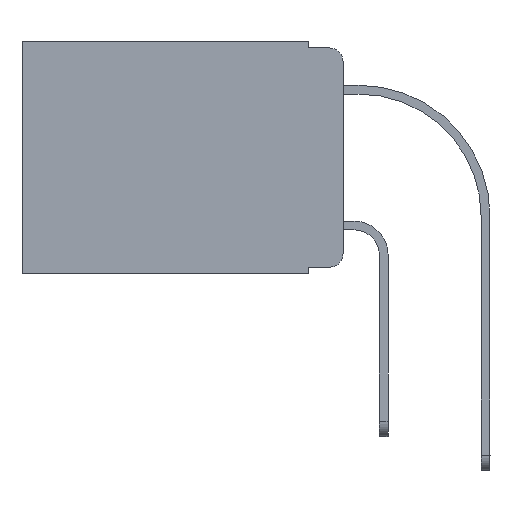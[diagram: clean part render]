
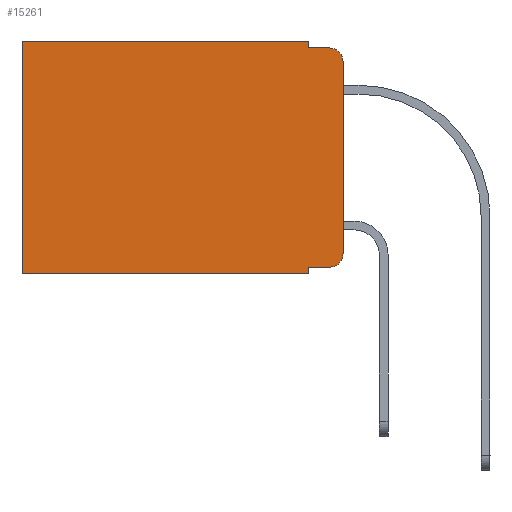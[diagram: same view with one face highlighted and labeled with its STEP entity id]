
A CAD part, left-side view. The second image highlights one B-rep face of the part: STEP entity #15261.
In plain terms, the highlighted planar face has unit normal (-1, 0, 0).
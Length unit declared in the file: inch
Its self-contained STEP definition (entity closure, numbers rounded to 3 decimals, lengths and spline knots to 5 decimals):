
#123 = CARTESIAN_POINT ( 'NONE',  ( 0.298, 0.02, -0.333 ) ) ;
#134 = CARTESIAN_POINT ( 'NONE',  ( 0.298, 0.051, -0.333 ) ) ;
#322 = CARTESIAN_POINT ( 'NONE',  ( 0.298, 0.051, -0.333 ) ) ;
#547 = VECTOR ( 'NONE', #4205, 39.37008 ) ;
#637 = EDGE_CURVE ( 'NONE', #14524, #1606, #16961, .T. ) ;
#685 = CARTESIAN_POINT ( 'NONE',  ( 0.298, 0.051, -0.01 ) ) ;
#919 = ORIENTED_EDGE ( 'NONE', *, *, #12089, .T. ) ;
#1377 = FACE_OUTER_BOUND ( 'NONE', #13782, .T. ) ;
#1388 = DIRECTION ( 'NONE',  ( 0., 0., -1. ) ) ;
#1590 = AXIS2_PLACEMENT_3D ( 'NONE', #2081, #9486, #15052 ) ;
#1606 = VERTEX_POINT ( 'NONE', #2224 ) ;
#1702 = CARTESIAN_POINT ( 'NONE',  ( 0.298, 0., 0. ) ) ;
#1849 = DIRECTION ( 'NONE',  ( 0., 1., 0. ) ) ;
#2081 = CARTESIAN_POINT ( 'NONE',  ( 0.298, 0.02, -0.03 ) ) ;
#2224 = CARTESIAN_POINT ( 'NONE',  ( 0.298, 0., -0.313 ) ) ;
#2403 = CARTESIAN_POINT ( 'NONE',  ( 0.298, 0.051, -0.01 ) ) ;
#2492 = AXIS2_PLACEMENT_3D ( 'NONE', #12650, #8907, #14354 ) ;
#2554 = VERTEX_POINT ( 'NONE', #14505 ) ;
#2789 = CARTESIAN_POINT ( 'NONE',  ( 0.298, 0.051, -0.343 ) ) ;
#2972 = DIRECTION ( 'NONE',  ( 0., 0., -1. ) ) ;
#3544 = ORIENTED_EDGE ( 'NONE', *, *, #9030, .T. ) ;
#3619 = LINE ( 'NONE', #14890, #21005 ) ;
#4083 = LINE ( 'NONE', #322, #547 ) ;
#4205 = DIRECTION ( 'NONE',  ( 0., -1., 0. ) ) ;
#4498 = ORIENTED_EDGE ( 'NONE', *, *, #12221, .F. ) ;
#4610 = VECTOR ( 'NONE', #21935, 39.37008 ) ;
#5077 = EDGE_CURVE ( 'NONE', #14524, #10999, #12043, .T. ) ;
#5282 = LINE ( 'NONE', #8964, #4610 ) ;
#5606 = CARTESIAN_POINT ( 'NONE',  ( 0.298, 0.051, 0. ) ) ;
#6018 = ORIENTED_EDGE ( 'NONE', *, *, #15777, .T. ) ;
#6424 = ORIENTED_EDGE ( 'NONE', *, *, #5077, .T. ) ;
#6554 = ORIENTED_EDGE ( 'NONE', *, *, #15941, .F. ) ;
#6641 = LINE ( 'NONE', #685, #23034 ) ;
#6961 = PLANE ( 'NONE',  #2492 ) ;
#7738 = VERTEX_POINT ( 'NONE', #134 ) ;
#8227 = DIRECTION ( 'NONE',  ( 0., 1., 0. ) ) ;
#8481 = VERTEX_POINT ( 'NONE', #22375 ) ;
#8907 = DIRECTION ( 'NONE',  ( 1., 0., 0. ) ) ;
#8964 = CARTESIAN_POINT ( 'NONE',  ( 0.298, 0.051, 0. ) ) ;
#9030 = EDGE_CURVE ( 'NONE', #11075, #2554, #16280, .T. ) ;
#9145 = CARTESIAN_POINT ( 'NONE',  ( 0.298, 0., 0. ) ) ;
#9486 = DIRECTION ( 'NONE',  ( -1., 0., 0. ) ) ;
#9660 = AXIS2_PLACEMENT_3D ( 'NONE', #12299, #19598, #2972 ) ;
#10999 = VERTEX_POINT ( 'NONE', #21644 ) ;
#11016 = DIRECTION ( 'NONE',  ( 0., 0., -1. ) ) ;
#11075 = VERTEX_POINT ( 'NONE', #5606 ) ;
#11209 = VECTOR ( 'NONE', #1388, 39.37008 ) ;
#11572 = VERTEX_POINT ( 'NONE', #123 ) ;
#11974 = DIRECTION ( 'NONE',  ( 0., -1., 0. ) ) ;
#12043 = CIRCLE ( 'NONE', #1590, 0.02 ) ;
#12089 = EDGE_CURVE ( 'NONE', #11572, #1606, #16243, .T. ) ;
#12100 = CARTESIAN_POINT ( 'NONE',  ( 0.298, 0., -0.343 ) ) ;
#12221 = EDGE_CURVE ( 'NONE', #7738, #19023, #21773, .T. ) ;
#12299 = CARTESIAN_POINT ( 'NONE',  ( 0.298, 0.02, -0.313 ) ) ;
#12377 = CARTESIAN_POINT ( 'NONE',  ( 0.298, 0., -0.03 ) ) ;
#12650 = CARTESIAN_POINT ( 'NONE',  ( 0.298, 0., 0. ) ) ;
#12701 = ORIENTED_EDGE ( 'NONE', *, *, #637, .F. ) ;
#13782 = EDGE_LOOP ( 'NONE', ( #12701, #6424, #16086, #17367, #3544, #22771, #6554, #4498, #6018, #919 ) ) ;
#14354 = DIRECTION ( 'NONE',  ( 0., 0., -1. ) ) ;
#14505 = CARTESIAN_POINT ( 'NONE',  ( 0.298, 0.473, 0. ) ) ;
#14524 = VERTEX_POINT ( 'NONE', #12377 ) ;
#14890 = CARTESIAN_POINT ( 'NONE',  ( 0.298, 0.473, 0. ) ) ;
#15052 = DIRECTION ( 'NONE',  ( 0., 0., -1. ) ) ;
#15261 = ADVANCED_FACE ( 'NONE', ( #1377 ), #6961, .F. ) ;
#15679 = VECTOR ( 'NONE', #8227, 39.37008 ) ;
#15777 = EDGE_CURVE ( 'NONE', #7738, #11572, #4083, .T. ) ;
#15862 = EDGE_CURVE ( 'NONE', #23822, #10999, #6641, .T. ) ;
#15941 = EDGE_CURVE ( 'NONE', #19023, #8481, #22907, .T. ) ;
#16086 = ORIENTED_EDGE ( 'NONE', *, *, #15862, .F. ) ;
#16243 = CIRCLE ( 'NONE', #9660, 0.02 ) ;
#16280 = LINE ( 'NONE', #9145, #23679 ) ;
#16961 = LINE ( 'NONE', #1702, #18557 ) ;
#17367 = ORIENTED_EDGE ( 'NONE', *, *, #20531, .F. ) ;
#18557 = VECTOR ( 'NONE', #20272, 39.37008 ) ;
#19023 = VERTEX_POINT ( 'NONE', #2789 ) ;
#19598 = DIRECTION ( 'NONE',  ( -1., 0., 0. ) ) ;
#20208 = CARTESIAN_POINT ( 'NONE',  ( 0.298, 0.051, 0. ) ) ;
#20272 = DIRECTION ( 'NONE',  ( 0., 0., -1. ) ) ;
#20531 = EDGE_CURVE ( 'NONE', #11075, #23822, #5282, .T. ) ;
#21005 = VECTOR ( 'NONE', #11016, 39.37008 ) ;
#21644 = CARTESIAN_POINT ( 'NONE',  ( 0.298, 0.02, -0.01 ) ) ;
#21773 = LINE ( 'NONE', #20208, #11209 ) ;
#21935 = DIRECTION ( 'NONE',  ( 0., 0., -1. ) ) ;
#22375 = CARTESIAN_POINT ( 'NONE',  ( 0.298, 0.473, -0.343 ) ) ;
#22771 = ORIENTED_EDGE ( 'NONE', *, *, #23649, .T. ) ;
#22907 = LINE ( 'NONE', #12100, #15679 ) ;
#23034 = VECTOR ( 'NONE', #11974, 39.37008 ) ;
#23649 = EDGE_CURVE ( 'NONE', #2554, #8481, #3619, .T. ) ;
#23679 = VECTOR ( 'NONE', #1849, 39.37008 ) ;
#23822 = VERTEX_POINT ( 'NONE', #2403 ) ;
